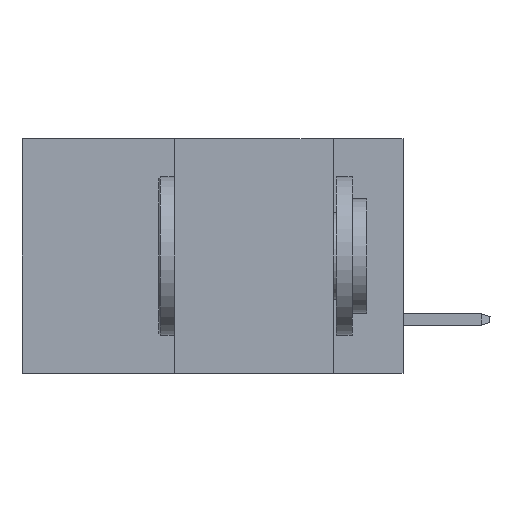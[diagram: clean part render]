
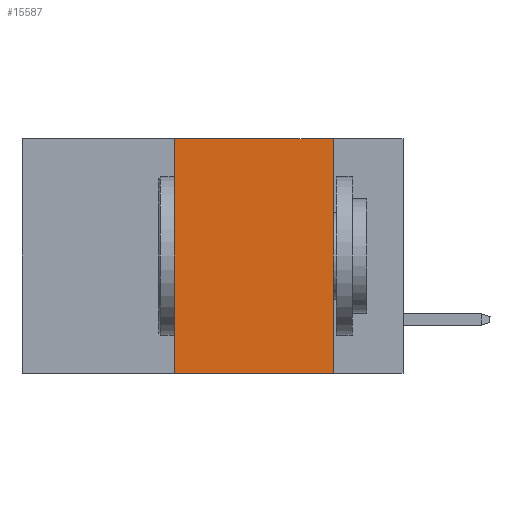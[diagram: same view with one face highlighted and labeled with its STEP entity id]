
A CAD part, left-side view. The second image highlights one B-rep face of the part: STEP entity #15587.
In plain terms, the highlighted planar face has unit normal (-1, 0, 0).
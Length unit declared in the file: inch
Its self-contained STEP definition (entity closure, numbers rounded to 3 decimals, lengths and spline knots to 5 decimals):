
#1017 = VERTEX_POINT ( 'NONE', #25082 ) ;
#2171 = VERTEX_POINT ( 'NONE', #11618 ) ;
#2811 = ORIENTED_EDGE ( 'NONE', *, *, #15119, .T. ) ;
#3294 = CARTESIAN_POINT ( 'NONE',  ( 0., 0.6, -0.37 ) ) ;
#3453 = VECTOR ( 'NONE', #3636, 39.37008 ) ;
#3636 = DIRECTION ( 'NONE',  ( 0., 0., 1. ) ) ;
#4237 = CARTESIAN_POINT ( 'NONE',  ( 0., 0.6, 0. ) ) ;
#6471 = EDGE_CURVE ( 'NONE', #2171, #1017, #27433, .T. ) ;
#6783 = VECTOR ( 'NONE', #12890, 39.37008 ) ;
#7012 = ORIENTED_EDGE ( 'NONE', *, *, #18901, .F. ) ;
#8285 = VECTOR ( 'NONE', #9189, 39.37008 ) ;
#9189 = DIRECTION ( 'NONE',  ( 0., -1., 0. ) ) ;
#10512 = CARTESIAN_POINT ( 'NONE',  ( 0., 0.11, 0. ) ) ;
#11521 = VERTEX_POINT ( 'NONE', #23327 ) ;
#11618 = CARTESIAN_POINT ( 'NONE',  ( 0., 0.36, -0.37 ) ) ;
#12340 = FACE_OUTER_BOUND ( 'NONE', #20454, .T. ) ;
#12890 = DIRECTION ( 'NONE',  ( 0., 0., -1. ) ) ;
#13205 = LINE ( 'NONE', #4237, #8285 ) ;
#14900 = PLANE ( 'NONE',  #16985 ) ;
#15119 = EDGE_CURVE ( 'NONE', #2171, #11521, #18659, .T. ) ;
#15587 = ADVANCED_FACE ( 'NONE', ( #12340 ), #14900, .F. ) ;
#16981 = VERTEX_POINT ( 'NONE', #10512 ) ;
#16985 = AXIS2_PLACEMENT_3D ( 'NONE', #18907, #23438, #27595 ) ;
#17205 = EDGE_CURVE ( 'NONE', #1017, #16981, #13205, .T. ) ;
#17764 = LINE ( 'NONE', #20003, #6783 ) ;
#18248 = DIRECTION ( 'NONE',  ( 0., -1., 0. ) ) ;
#18659 = LINE ( 'NONE', #3294, #19193 ) ;
#18901 = EDGE_CURVE ( 'NONE', #16981, #11521, #17764, .T. ) ;
#18907 = CARTESIAN_POINT ( 'NONE',  ( 0., 0.6, 0. ) ) ;
#19193 = VECTOR ( 'NONE', #18248, 39.37008 ) ;
#20003 = CARTESIAN_POINT ( 'NONE',  ( 0., 0.11, 0. ) ) ;
#20454 = EDGE_LOOP ( 'NONE', ( #7012, #23700, #22319, #2811 ) ) ;
#22319 = ORIENTED_EDGE ( 'NONE', *, *, #6471, .F. ) ;
#23327 = CARTESIAN_POINT ( 'NONE',  ( 0., 0.11, -0.37 ) ) ;
#23438 = DIRECTION ( 'NONE',  ( 1., 0., 0. ) ) ;
#23700 = ORIENTED_EDGE ( 'NONE', *, *, #17205, .F. ) ;
#25082 = CARTESIAN_POINT ( 'NONE',  ( 0., 0.36, 0. ) ) ;
#25693 = CARTESIAN_POINT ( 'NONE',  ( 0., 0.36, 0. ) ) ;
#27433 = LINE ( 'NONE', #25693, #3453 ) ;
#27595 = DIRECTION ( 'NONE',  ( 0., 0., -1. ) ) ;
